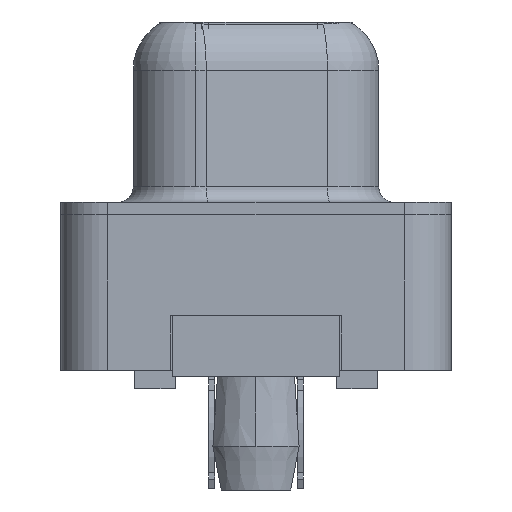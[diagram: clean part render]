
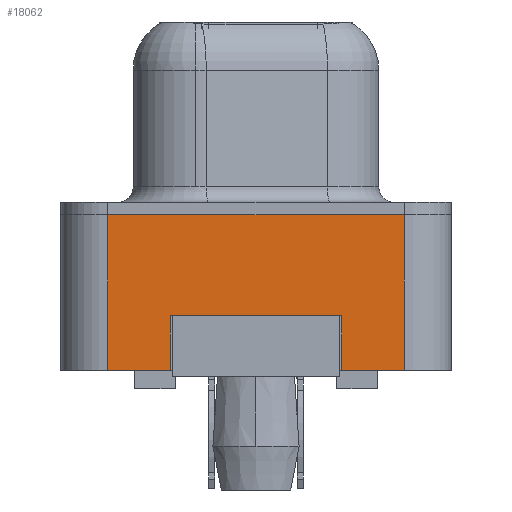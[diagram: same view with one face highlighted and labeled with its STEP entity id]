
A CAD part, left-side view. The second image highlights one B-rep face of the part: STEP entity #18062.
In plain terms, the highlighted planar face has unit normal (-1, 0, 0).
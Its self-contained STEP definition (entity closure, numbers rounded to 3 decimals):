
#501 = ORIENTED_EDGE ( 'NONE', *, *, #10026, .T. ) ;
#1736 = EDGE_CURVE ( 'NONE', #14162, #9845, #8119, .T. ) ;
#1778 = CARTESIAN_POINT ( 'NONE',  ( -2.995, 4.775, -5. ) ) ;
#2012 = VECTOR ( 'NONE', #15980, 1000. ) ;
#2436 = VERTEX_POINT ( 'NONE', #17339 ) ;
#2474 = VECTOR ( 'NONE', #10392, 1000. ) ;
#2713 = LINE ( 'NONE', #13010, #17952 ) ;
#2772 = LINE ( 'NONE', #11321, #15602 ) ;
#2894 = ORIENTED_EDGE ( 'NONE', *, *, #4841, .F. ) ;
#3471 = LINE ( 'NONE', #20125, #3606 ) ;
#3606 = VECTOR ( 'NONE', #9936, 1000. ) ;
#4147 = LINE ( 'NONE', #4262, #2012 ) ;
#4250 = LINE ( 'NONE', #10610, #20323 ) ;
#4262 = CARTESIAN_POINT ( 'NONE',  ( -2.995, -4.775, -5. ) ) ;
#4541 = CARTESIAN_POINT ( 'NONE',  ( -2.995, -4.775, -5. ) ) ;
#4576 = DIRECTION ( 'NONE',  ( 0., 0., 1. ) ) ;
#4841 = EDGE_CURVE ( 'NONE', #20975, #20991, #2772, .T. ) ;
#5620 = ORIENTED_EDGE ( 'NONE', *, *, #19992, .T. ) ;
#6302 = EDGE_CURVE ( 'NONE', #12459, #2436, #4147, .T. ) ;
#6659 = ORIENTED_EDGE ( 'NONE', *, *, #16215, .F. ) ;
#7325 = DIRECTION ( 'NONE',  ( 0., 1., 0. ) ) ;
#7987 = CARTESIAN_POINT ( 'NONE',  ( -2.995, -2.75, -3.25 ) ) ;
#8095 = LINE ( 'NONE', #9729, #18318 ) ;
#8119 = LINE ( 'NONE', #14586, #13262 ) ;
#8189 = AXIS2_PLACEMENT_3D ( 'NONE', #4541, #21404, #18022 ) ;
#8471 = CARTESIAN_POINT ( 'NONE',  ( -2.995, -4.775, -5. ) ) ;
#8887 = ORIENTED_EDGE ( 'NONE', *, *, #10453, .F. ) ;
#9351 = PLANE ( 'NONE',  #8189 ) ;
#9444 = VERTEX_POINT ( 'NONE', #1778 ) ;
#9729 = CARTESIAN_POINT ( 'NONE',  ( -2.995, -4.775, -5. ) ) ;
#9745 = CARTESIAN_POINT ( 'NONE',  ( -2.995, -2.75, -5. ) ) ;
#9845 = VERTEX_POINT ( 'NONE', #9745 ) ;
#9936 = DIRECTION ( 'NONE',  ( 0., -1., 0. ) ) ;
#10026 = EDGE_CURVE ( 'NONE', #9845, #12459, #12042, .T. ) ;
#10039 = ORIENTED_EDGE ( 'NONE', *, *, #6302, .T. ) ;
#10392 = DIRECTION ( 'NONE',  ( 0., -1., 0. ) ) ;
#10453 = EDGE_CURVE ( 'NONE', #14162, #20975, #4250, .T. ) ;
#10480 = ORIENTED_EDGE ( 'NONE', *, *, #15942, .F. ) ;
#10610 = CARTESIAN_POINT ( 'NONE',  ( -2.995, 2.75, -3.25 ) ) ;
#10784 = CARTESIAN_POINT ( 'NONE',  ( -2.995, 2.75, -3.25 ) ) ;
#11304 = DIRECTION ( 'NONE',  ( 0., 0., -1. ) ) ;
#11321 = CARTESIAN_POINT ( 'NONE',  ( -2.995, 2.75, -3.25 ) ) ;
#12042 = LINE ( 'NONE', #18737, #2474 ) ;
#12459 = VERTEX_POINT ( 'NONE', #8471 ) ;
#12539 = CARTESIAN_POINT ( 'NONE',  ( -2.995, 4.775, 0. ) ) ;
#13010 = CARTESIAN_POINT ( 'NONE',  ( -2.995, 4.775, -5. ) ) ;
#13077 = DIRECTION ( 'NONE',  ( 0., 0., -1. ) ) ;
#13262 = VECTOR ( 'NONE', #11304, 1000. ) ;
#13439 = ORIENTED_EDGE ( 'NONE', *, *, #1736, .T. ) ;
#14162 = VERTEX_POINT ( 'NONE', #7987 ) ;
#14586 = CARTESIAN_POINT ( 'NONE',  ( -2.995, -2.75, -3.25 ) ) ;
#15602 = VECTOR ( 'NONE', #13077, 1000. ) ;
#15942 = EDGE_CURVE ( 'NONE', #9444, #20939, #2713, .T. ) ;
#15980 = DIRECTION ( 'NONE',  ( 0., 0., 1. ) ) ;
#16215 = EDGE_CURVE ( 'NONE', #20939, #2436, #3471, .T. ) ;
#16324 = DIRECTION ( 'NONE',  ( 0., -1., 0. ) ) ;
#17339 = CARTESIAN_POINT ( 'NONE',  ( -2.995, -4.775, 0. ) ) ;
#17952 = VECTOR ( 'NONE', #4576, 1000. ) ;
#18022 = DIRECTION ( 'NONE',  ( 0., 0., 1. ) ) ;
#18062 = ADVANCED_FACE ( 'NONE', ( #19875 ), #9351, .T. ) ;
#18318 = VECTOR ( 'NONE', #16324, 1000. ) ;
#18737 = CARTESIAN_POINT ( 'NONE',  ( -2.995, -4.775, -5. ) ) ;
#19135 = EDGE_LOOP ( 'NONE', ( #13439, #501, #10039, #6659, #10480, #5620, #2894, #8887 ) ) ;
#19875 = FACE_OUTER_BOUND ( 'NONE', #19135, .T. ) ;
#19992 = EDGE_CURVE ( 'NONE', #9444, #20991, #8095, .T. ) ;
#20125 = CARTESIAN_POINT ( 'NONE',  ( -2.995, -4.775, 0. ) ) ;
#20323 = VECTOR ( 'NONE', #7325, 1000. ) ;
#20939 = VERTEX_POINT ( 'NONE', #12539 ) ;
#20970 = CARTESIAN_POINT ( 'NONE',  ( -2.995, 2.75, -5. ) ) ;
#20975 = VERTEX_POINT ( 'NONE', #10784 ) ;
#20991 = VERTEX_POINT ( 'NONE', #20970 ) ;
#21404 = DIRECTION ( 'NONE',  ( -1., 0., 0. ) ) ;
